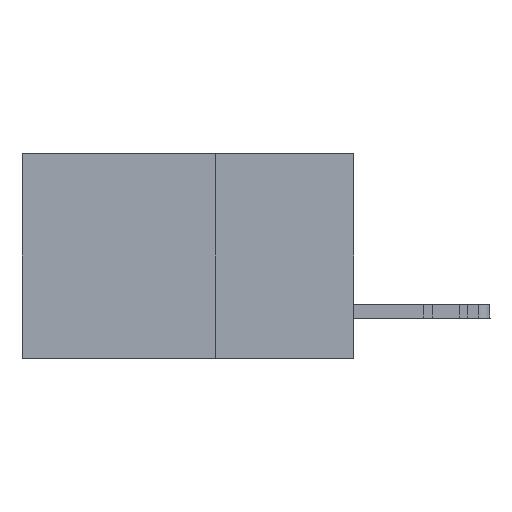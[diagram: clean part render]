
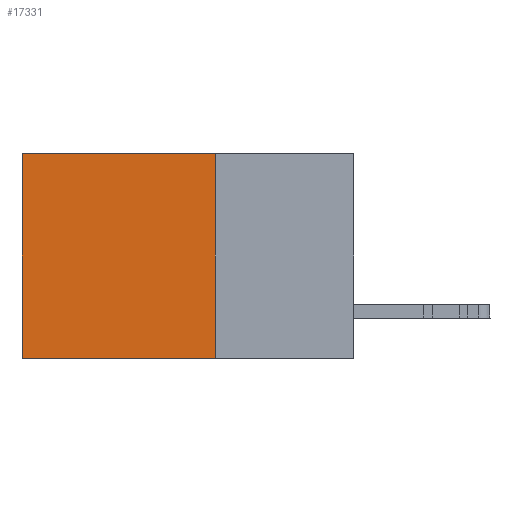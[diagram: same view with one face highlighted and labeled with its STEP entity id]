
A CAD part, left-side view. The second image highlights one B-rep face of the part: STEP entity #17331.
In plain terms, the highlighted planar face has unit normal (-1, 0, 0).
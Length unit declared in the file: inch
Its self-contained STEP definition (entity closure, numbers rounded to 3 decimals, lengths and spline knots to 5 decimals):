
#898 = DIRECTION ( 'NONE',  ( 0., 1., 0. ) ) ;
#2411 = VECTOR ( 'NONE', #24463, 39.37008 ) ;
#2797 = DIRECTION ( 'NONE',  ( 0., 0., -1. ) ) ;
#6261 = VECTOR ( 'NONE', #25117, 39.37008 ) ;
#7314 = VERTEX_POINT ( 'NONE', #19702 ) ;
#10627 = DIRECTION ( 'NONE',  ( 1., 0., 0. ) ) ;
#10764 = CARTESIAN_POINT ( 'NONE',  ( 0.2875, 0.25, 0. ) ) ;
#11793 = LINE ( 'NONE', #35310, #6261 ) ;
#11953 = EDGE_CURVE ( 'NONE', #7314, #12395, #11793, .T. ) ;
#12006 = FACE_OUTER_BOUND ( 'NONE', #29754, .T. ) ;
#12395 = VERTEX_POINT ( 'NONE', #28686 ) ;
#14644 = DIRECTION ( 'NONE',  ( 0., 0., -1. ) ) ;
#15389 = VECTOR ( 'NONE', #898, 39.37008 ) ;
#17331 = ADVANCED_FACE ( 'NONE', ( #12006 ), #28747, .F. ) ;
#18193 = LINE ( 'NONE', #45079, #27027 ) ;
#18376 = CARTESIAN_POINT ( 'NONE',  ( 0.2875, 0.6, 0. ) ) ;
#19702 = CARTESIAN_POINT ( 'NONE',  ( 0.2875, 0.25, 0. ) ) ;
#20815 = EDGE_CURVE ( 'NONE', #12395, #38757, #36715, .T. ) ;
#23854 = AXIS2_PLACEMENT_3D ( 'NONE', #10764, #10627, #14644 ) ;
#24463 = DIRECTION ( 'NONE',  ( 0., 1., 0. ) ) ;
#25010 = CARTESIAN_POINT ( 'NONE',  ( 0.2875, 0.25, -0.37 ) ) ;
#25117 = DIRECTION ( 'NONE',  ( 0., 0., -1. ) ) ;
#27027 = VECTOR ( 'NONE', #2797, 39.37008 ) ;
#27482 = ORIENTED_EDGE ( 'NONE', *, *, #20815, .F. ) ;
#27499 = CARTESIAN_POINT ( 'NONE',  ( 0.2875, 0.6, -0.37 ) ) ;
#28686 = CARTESIAN_POINT ( 'NONE',  ( 0.2875, 0.25, -0.37 ) ) ;
#28747 = PLANE ( 'NONE',  #23854 ) ;
#29754 = EDGE_LOOP ( 'NONE', ( #32163, #27482, #45648, #41811 ) ) ;
#32163 = ORIENTED_EDGE ( 'NONE', *, *, #44245, .T. ) ;
#35310 = CARTESIAN_POINT ( 'NONE',  ( 0.2875, 0.25, 0. ) ) ;
#36715 = LINE ( 'NONE', #25010, #2411 ) ;
#37008 = VERTEX_POINT ( 'NONE', #18376 ) ;
#37479 = LINE ( 'NONE', #39673, #15389 ) ;
#38757 = VERTEX_POINT ( 'NONE', #27499 ) ;
#39673 = CARTESIAN_POINT ( 'NONE',  ( 0.2875, 0.25, 0. ) ) ;
#41529 = EDGE_CURVE ( 'NONE', #7314, #37008, #37479, .T. ) ;
#41811 = ORIENTED_EDGE ( 'NONE', *, *, #41529, .T. ) ;
#44245 = EDGE_CURVE ( 'NONE', #37008, #38757, #18193, .T. ) ;
#45079 = CARTESIAN_POINT ( 'NONE',  ( 0.2875, 0.6, 0. ) ) ;
#45648 = ORIENTED_EDGE ( 'NONE', *, *, #11953, .F. ) ;
